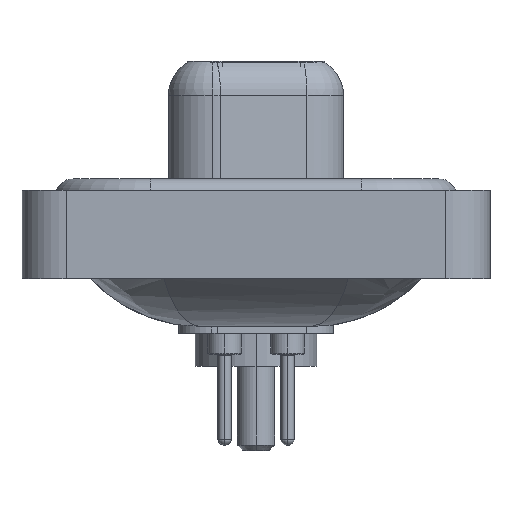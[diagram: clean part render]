
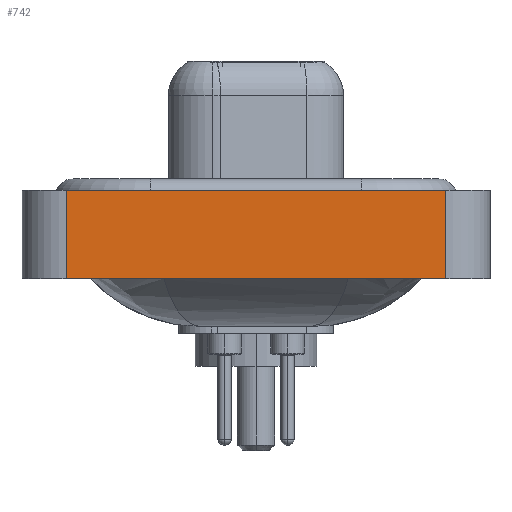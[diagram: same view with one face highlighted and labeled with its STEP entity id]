
A CAD part, left-side view. The second image highlights one B-rep face of the part: STEP entity #742.
In plain terms, the highlighted planar face has unit normal (-1, 0, 0).
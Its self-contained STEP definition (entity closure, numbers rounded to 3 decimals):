
#250 = CARTESIAN_POINT ( 'NONE',  ( -7.35, -8.55, 0.4 ) ) ;
#341 = ORIENTED_EDGE ( 'NONE', *, *, #17238, .T. ) ;
#742 = ADVANCED_FACE ( 'NONE', ( #23069 ), #3007, .T. ) ;
#3007 = PLANE ( 'NONE',  #23721 ) ;
#3018 = DIRECTION ( 'NONE',  ( 0., 0., 1. ) ) ;
#3172 = CARTESIAN_POINT ( 'NONE',  ( -7.35, 8.55, -3.6 ) ) ;
#5034 = CARTESIAN_POINT ( 'NONE',  ( -7.35, 8.55, 0.4 ) ) ;
#5282 = LINE ( 'NONE', #14912, #11530 ) ;
#5917 = ORIENTED_EDGE ( 'NONE', *, *, #22677, .F. ) ;
#6627 = CARTESIAN_POINT ( 'NONE',  ( -7.35, 8.55, -3.6 ) ) ;
#7026 = CARTESIAN_POINT ( 'NONE',  ( -7.35, -8.55, -3.6 ) ) ;
#9434 = EDGE_CURVE ( 'NONE', #20270, #16013, #25084, .T. ) ;
#9892 = DIRECTION ( 'NONE',  ( 0., -1., 0. ) ) ;
#10706 = VERTEX_POINT ( 'NONE', #5034 ) ;
#10788 = VECTOR ( 'NONE', #25849, 1000. ) ;
#10896 = ORIENTED_EDGE ( 'NONE', *, *, #9434, .T. ) ;
#10968 = LINE ( 'NONE', #6627, #15933 ) ;
#11530 = VECTOR ( 'NONE', #3018, 1000. ) ;
#11846 = ORIENTED_EDGE ( 'NONE', *, *, #13029, .F. ) ;
#12802 = DIRECTION ( 'NONE',  ( -1., 0., 0. ) ) ;
#13029 = EDGE_CURVE ( 'NONE', #20270, #10706, #10968, .T. ) ;
#13188 = CARTESIAN_POINT ( 'NONE',  ( -7.35, -8.55, -3.6 ) ) ;
#14912 = CARTESIAN_POINT ( 'NONE',  ( -7.35, -8.55, -3.6 ) ) ;
#15433 = CARTESIAN_POINT ( 'NONE',  ( -7.35, -8.55, -3.6 ) ) ;
#15660 = CARTESIAN_POINT ( 'NONE',  ( -7.35, -8.55, 0.4 ) ) ;
#15933 = VECTOR ( 'NONE', #22697, 1000. ) ;
#16013 = VERTEX_POINT ( 'NONE', #15433 ) ;
#16763 = DIRECTION ( 'NONE',  ( 0., 0., 1. ) ) ;
#17238 = EDGE_CURVE ( 'NONE', #16013, #19040, #5282, .T. ) ;
#18574 = EDGE_LOOP ( 'NONE', ( #341, #5917, #11846, #10896 ) ) ;
#19040 = VERTEX_POINT ( 'NONE', #15660 ) ;
#19911 = LINE ( 'NONE', #250, #23523 ) ;
#20270 = VERTEX_POINT ( 'NONE', #3172 ) ;
#22677 = EDGE_CURVE ( 'NONE', #10706, #19040, #19911, .T. ) ;
#22697 = DIRECTION ( 'NONE',  ( 0., 0., 1. ) ) ;
#23069 = FACE_OUTER_BOUND ( 'NONE', #18574, .T. ) ;
#23523 = VECTOR ( 'NONE', #9892, 1000. ) ;
#23721 = AXIS2_PLACEMENT_3D ( 'NONE', #13188, #12802, #16763 ) ;
#25084 = LINE ( 'NONE', #7026, #10788 ) ;
#25849 = DIRECTION ( 'NONE',  ( 0., -1., 0. ) ) ;
